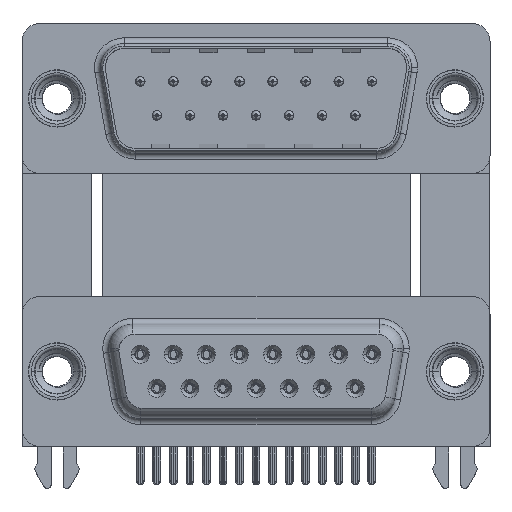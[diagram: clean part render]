
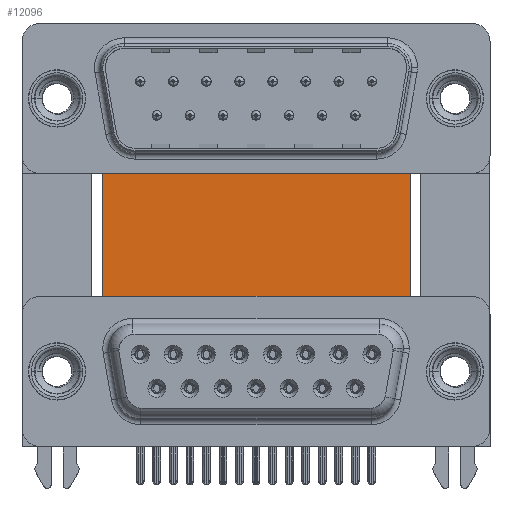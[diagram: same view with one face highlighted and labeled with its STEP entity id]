
A CAD part, top view. The second image highlights one B-rep face of the part: STEP entity #12096.
In plain terms, the highlighted planar face has unit normal (0, 0, 1).
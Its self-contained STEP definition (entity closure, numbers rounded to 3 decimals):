
#1078 = EDGE_CURVE ( 'NONE', #42888, #31185, #32159, .T. ) ;
#1121 = VERTEX_POINT ( 'NONE', #29105 ) ;
#1299 = LINE ( 'NONE', #12385, #15813 ) ;
#3608 = DIRECTION ( 'NONE',  ( 0., -1., 0. ) ) ;
#6651 = ORIENTED_EDGE ( 'NONE', *, *, #7671, .F. ) ;
#7671 = EDGE_CURVE ( 'NONE', #27300, #1121, #1299, .T. ) ;
#7840 = ORIENTED_EDGE ( 'NONE', *, *, #1078, .T. ) ;
#8058 = CARTESIAN_POINT ( 'NONE',  ( 3.79, 16.585, -12. ) ) ;
#8770 = VECTOR ( 'NONE', #12516, 1000. ) ;
#12096 = ADVANCED_FACE ( 'NONE', ( #21434 ), #32293, .F. ) ;
#12385 = CARTESIAN_POINT ( 'NONE',  ( 3.79, 16.585, -12. ) ) ;
#12516 = DIRECTION ( 'NONE',  ( 0., -1., 0. ) ) ;
#13453 = CARTESIAN_POINT ( 'NONE',  ( 3.79, -3.735, -12. ) ) ;
#14348 = DIRECTION ( 'NONE',  ( 0., 0., -1. ) ) ;
#15699 = DIRECTION ( 'NONE',  ( 1., 0., 0. ) ) ;
#15813 = VECTOR ( 'NONE', #15699, 1000. ) ;
#16799 = EDGE_CURVE ( 'NONE', #1121, #31185, #21091, .T. ) ;
#18509 = CARTESIAN_POINT ( 'NONE',  ( 29.58, -3.735, -12. ) ) ;
#20689 = VECTOR ( 'NONE', #3608, 1000. ) ;
#21091 = LINE ( 'NONE', #39283, #20689 ) ;
#21434 = FACE_OUTER_BOUND ( 'NONE', #27473, .T. ) ;
#21496 = EDGE_CURVE ( 'NONE', #27300, #42888, #22466, .T. ) ;
#22302 = ORIENTED_EDGE ( 'NONE', *, *, #21496, .T. ) ;
#22466 = LINE ( 'NONE', #8058, #8770 ) ;
#24923 = AXIS2_PLACEMENT_3D ( 'NONE', #39858, #14348, #28774 ) ;
#25335 = DIRECTION ( 'NONE',  ( 1., 0., 0. ) ) ;
#27300 = VERTEX_POINT ( 'NONE', #30372 ) ;
#27473 = EDGE_LOOP ( 'NONE', ( #7840, #41121, #6651, #22302 ) ) ;
#28774 = DIRECTION ( 'NONE',  ( -1., 0., 0. ) ) ;
#29105 = CARTESIAN_POINT ( 'NONE',  ( 29.58, 16.585, -12. ) ) ;
#30372 = CARTESIAN_POINT ( 'NONE',  ( 3.79, 16.585, -12. ) ) ;
#31185 = VERTEX_POINT ( 'NONE', #18509 ) ;
#32159 = LINE ( 'NONE', #36426, #44394 ) ;
#32293 = PLANE ( 'NONE',  #24923 ) ;
#36426 = CARTESIAN_POINT ( 'NONE',  ( 3.79, -3.735, -12. ) ) ;
#39283 = CARTESIAN_POINT ( 'NONE',  ( 29.58, 16.585, -12. ) ) ;
#39858 = CARTESIAN_POINT ( 'NONE',  ( 3.79, 16.585, -12. ) ) ;
#41121 = ORIENTED_EDGE ( 'NONE', *, *, #16799, .F. ) ;
#42888 = VERTEX_POINT ( 'NONE', #13453 ) ;
#44394 = VECTOR ( 'NONE', #25335, 1000. ) ;
